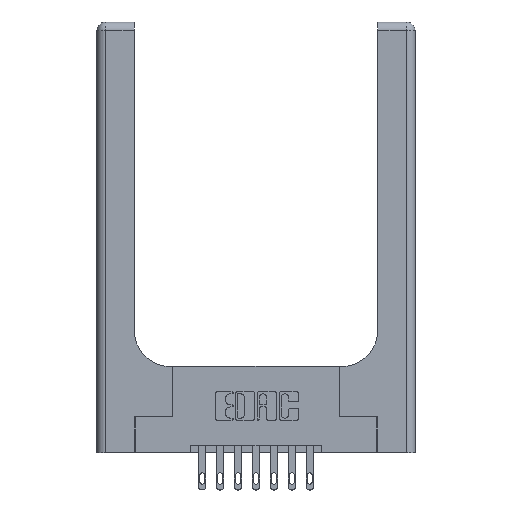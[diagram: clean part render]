
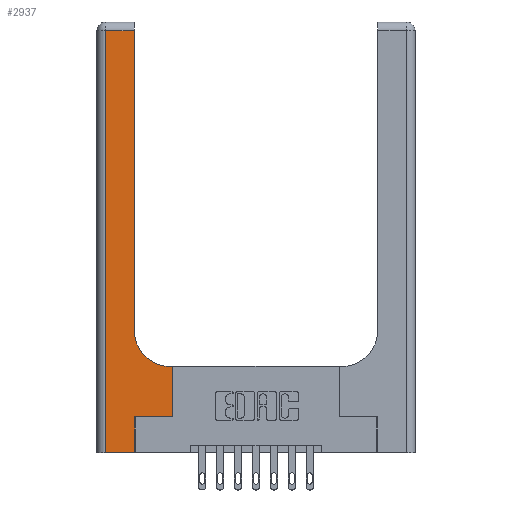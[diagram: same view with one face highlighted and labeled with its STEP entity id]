
A CAD part, top view. The second image highlights one B-rep face of the part: STEP entity #2937.
In plain terms, the highlighted planar face has unit normal (0, 0, 1).
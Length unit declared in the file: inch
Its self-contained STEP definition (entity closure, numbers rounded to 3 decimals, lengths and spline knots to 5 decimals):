
#70 = FACE_OUTER_BOUND ( 'NONE', #2662, .T. ) ;
#322 = VECTOR ( 'NONE', #2831, 39.37008 ) ;
#338 = ORIENTED_EDGE ( 'NONE', *, *, #13693, .T. ) ;
#841 = VECTOR ( 'NONE', #12476, 39.37008 ) ;
#900 = LINE ( 'NONE', #4061, #4901 ) ;
#904 = VERTEX_POINT ( 'NONE', #5534 ) ;
#1229 = EDGE_CURVE ( 'NONE', #6087, #11212, #3108, .T. ) ;
#1345 = CARTESIAN_POINT ( 'NONE',  ( 0.26, 0.6, 0.37 ) ) ;
#1543 = AXIS2_PLACEMENT_3D ( 'NONE', #14038, #3546, #3680 ) ;
#2055 = LINE ( 'NONE', #3331, #841 ) ;
#2172 = CARTESIAN_POINT ( 'NONE',  ( 0.265, 0., 0.37 ) ) ;
#2662 = EDGE_LOOP ( 'NONE', ( #3110, #7725, #338, #9557, #3191, #14044, #13429, #5599, #6537 ) ) ;
#2831 = DIRECTION ( 'NONE',  ( 0., 1., 0. ) ) ;
#2937 = ADVANCED_FACE ( 'NONE', ( #70 ), #9397, .F. ) ;
#3099 = CARTESIAN_POINT ( 'NONE',  ( 0.265, 0.25, 0.37 ) ) ;
#3108 = LINE ( 'NONE', #4378, #13350 ) ;
#3110 = ORIENTED_EDGE ( 'NONE', *, *, #9829, .T. ) ;
#3152 = VERTEX_POINT ( 'NONE', #2172 ) ;
#3191 = ORIENTED_EDGE ( 'NONE', *, *, #4854, .T. ) ;
#3331 = CARTESIAN_POINT ( 'NONE',  ( 0.265, 0.25, 0.37 ) ) ;
#3546 = DIRECTION ( 'NONE',  ( 0., 0., -1. ) ) ;
#3598 = CARTESIAN_POINT ( 'NONE',  ( 0.51, 0.85, 0.37 ) ) ;
#3680 = DIRECTION ( 'NONE',  ( -1., 0., 0. ) ) ;
#4061 = CARTESIAN_POINT ( 'NONE',  ( 0., 0., 0.37 ) ) ;
#4226 = LINE ( 'NONE', #12094, #14750 ) ;
#4378 = CARTESIAN_POINT ( 'NONE',  ( 0., 2.94, 0.37 ) ) ;
#4413 = VECTOR ( 'NONE', #6776, 39.37008 ) ;
#4670 = LINE ( 'NONE', #12471, #4413 ) ;
#4854 = EDGE_CURVE ( 'NONE', #3152, #11082, #7918, .T. ) ;
#4901 = VECTOR ( 'NONE', #10062, 39.37008 ) ;
#5126 = DIRECTION ( 'NONE',  ( 0., 1., 0. ) ) ;
#5312 = EDGE_CURVE ( 'NONE', #8278, #6909, #9731, .T. ) ;
#5355 = CARTESIAN_POINT ( 'NONE',  ( 0.265, 0., 0.37 ) ) ;
#5534 = CARTESIAN_POINT ( 'NONE',  ( 0.51, 0.6, 0.37 ) ) ;
#5599 = ORIENTED_EDGE ( 'NONE', *, *, #11295, .T. ) ;
#5638 = VERTEX_POINT ( 'NONE', #9504 ) ;
#5796 = CARTESIAN_POINT ( 'NONE',  ( 0.06, 2.94, 0.37 ) ) ;
#5978 = EDGE_CURVE ( 'NONE', #11082, #8278, #2055, .T. ) ;
#6087 = VERTEX_POINT ( 'NONE', #14053 ) ;
#6537 = ORIENTED_EDGE ( 'NONE', *, *, #11300, .T. ) ;
#6776 = DIRECTION ( 'NONE',  ( 0., -1., 0. ) ) ;
#6909 = VERTEX_POINT ( 'NONE', #12808 ) ;
#6985 = LINE ( 'NONE', #1345, #9517 ) ;
#7725 = ORIENTED_EDGE ( 'NONE', *, *, #1229, .T. ) ;
#7857 = AXIS2_PLACEMENT_3D ( 'NONE', #3598, #8184, #14018 ) ;
#7859 = DIRECTION ( 'NONE',  ( -1., 0., 0. ) ) ;
#7918 = LINE ( 'NONE', #5355, #11413 ) ;
#8184 = DIRECTION ( 'NONE',  ( 0., 0., -1. ) ) ;
#8278 = VERTEX_POINT ( 'NONE', #14302 ) ;
#9397 = PLANE ( 'NONE',  #1543 ) ;
#9504 = CARTESIAN_POINT ( 'NONE',  ( 0.06, 0., 0.37 ) ) ;
#9517 = VECTOR ( 'NONE', #11547, 39.37008 ) ;
#9557 = ORIENTED_EDGE ( 'NONE', *, *, #14065, .T. ) ;
#9731 = LINE ( 'NONE', #11984, #322 ) ;
#9829 = EDGE_CURVE ( 'NONE', #10332, #6087, #4226, .T. ) ;
#10062 = DIRECTION ( 'NONE',  ( 1., 0., 0. ) ) ;
#10078 = DIRECTION ( 'NONE',  ( 0., 1., 0. ) ) ;
#10332 = VERTEX_POINT ( 'NONE', #14180 ) ;
#11082 = VERTEX_POINT ( 'NONE', #3099 ) ;
#11212 = VERTEX_POINT ( 'NONE', #5796 ) ;
#11295 = EDGE_CURVE ( 'NONE', #6909, #904, #6985, .T. ) ;
#11300 = EDGE_CURVE ( 'NONE', #904, #10332, #11897, .T. ) ;
#11413 = VECTOR ( 'NONE', #10078, 39.37008 ) ;
#11547 = DIRECTION ( 'NONE',  ( -1., 0., 0. ) ) ;
#11897 = CIRCLE ( 'NONE', #7857, 0.25 ) ;
#11984 = CARTESIAN_POINT ( 'NONE',  ( 0.528, 0.25, 0.37 ) ) ;
#12094 = CARTESIAN_POINT ( 'NONE',  ( 0.26, 3., 0.37 ) ) ;
#12471 = CARTESIAN_POINT ( 'NONE',  ( 0.06, 3., 0.37 ) ) ;
#12476 = DIRECTION ( 'NONE',  ( 1., 0., 0. ) ) ;
#12808 = CARTESIAN_POINT ( 'NONE',  ( 0.528, 0.6, 0.37 ) ) ;
#13350 = VECTOR ( 'NONE', #7859, 39.37008 ) ;
#13429 = ORIENTED_EDGE ( 'NONE', *, *, #5312, .T. ) ;
#13693 = EDGE_CURVE ( 'NONE', #11212, #5638, #4670, .T. ) ;
#14018 = DIRECTION ( 'NONE',  ( 1., 0., 0. ) ) ;
#14038 = CARTESIAN_POINT ( 'NONE',  ( 0., 3., 0.37 ) ) ;
#14044 = ORIENTED_EDGE ( 'NONE', *, *, #5978, .T. ) ;
#14053 = CARTESIAN_POINT ( 'NONE',  ( 0.26, 2.94, 0.37 ) ) ;
#14065 = EDGE_CURVE ( 'NONE', #5638, #3152, #900, .T. ) ;
#14180 = CARTESIAN_POINT ( 'NONE',  ( 0.26, 0.85, 0.37 ) ) ;
#14302 = CARTESIAN_POINT ( 'NONE',  ( 0.528, 0.25, 0.37 ) ) ;
#14750 = VECTOR ( 'NONE', #5126, 39.37008 ) ;
